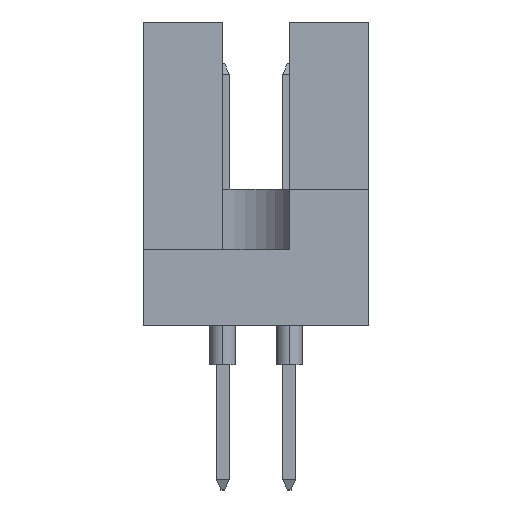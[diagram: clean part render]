
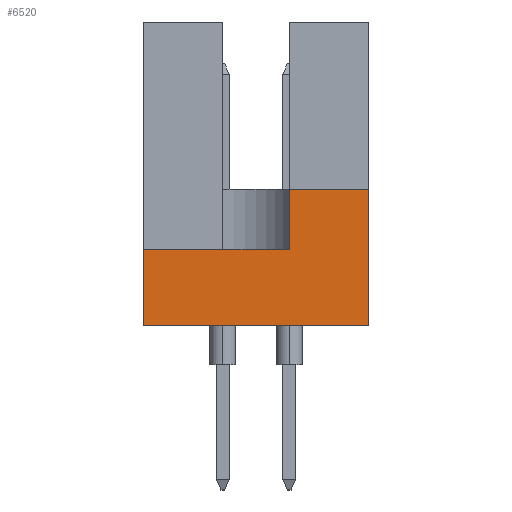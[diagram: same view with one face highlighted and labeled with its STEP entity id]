
A CAD part, left-side view. The second image highlights one B-rep face of the part: STEP entity #6520.
In plain terms, the highlighted planar face has unit normal (-1, 0, 0).
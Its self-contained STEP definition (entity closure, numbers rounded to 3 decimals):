
#75 = LINE ( 'NONE', #5244, #7016 ) ;
#217 = CARTESIAN_POINT ( 'NONE',  ( -47.5, -1.27, 2.9 ) ) ;
#599 = CARTESIAN_POINT ( 'NONE',  ( -47.5, -1.27, 19.02 ) ) ;
#619 = VECTOR ( 'NONE', #12354, 1000. ) ;
#737 = EDGE_LOOP ( 'NONE', ( #1978, #6213, #4580, #10751, #9131, #5655 ) ) ;
#951 = EDGE_CURVE ( 'NONE', #4590, #9276, #6410, .T. ) ;
#1071 = CARTESIAN_POINT ( 'NONE',  ( -47.5, 4.3, 0. ) ) ;
#1280 = DIRECTION ( 'NONE',  ( 1., 0., 0. ) ) ;
#1549 = LINE ( 'NONE', #3487, #9352 ) ;
#1978 = ORIENTED_EDGE ( 'NONE', *, *, #951, .F. ) ;
#2092 = PLANE ( 'NONE',  #5794 ) ;
#2777 = VECTOR ( 'NONE', #7641, 1000. ) ;
#3355 = DIRECTION ( 'NONE',  ( 0., 0., -1. ) ) ;
#3487 = CARTESIAN_POINT ( 'NONE',  ( -47.5, 4.3, 11.6 ) ) ;
#3809 = CARTESIAN_POINT ( 'NONE',  ( -47.5, -4.3, 5.2 ) ) ;
#4474 = DIRECTION ( 'NONE',  ( 0., 0., -1. ) ) ;
#4580 = ORIENTED_EDGE ( 'NONE', *, *, #7950, .T. ) ;
#4590 = VERTEX_POINT ( 'NONE', #7019 ) ;
#4821 = CARTESIAN_POINT ( 'NONE',  ( -47.5, -4.3, 0. ) ) ;
#5093 = EDGE_CURVE ( 'NONE', #9420, #11876, #5805, .T. ) ;
#5109 = VECTOR ( 'NONE', #11801, 1000. ) ;
#5244 = CARTESIAN_POINT ( 'NONE',  ( -47.5, 4.3, 2.9 ) ) ;
#5418 = EDGE_CURVE ( 'NONE', #10398, #9420, #1549, .T. ) ;
#5422 = DIRECTION ( 'NONE',  ( 0., -1., 0. ) ) ;
#5504 = LINE ( 'NONE', #9497, #619 ) ;
#5655 = ORIENTED_EDGE ( 'NONE', *, *, #10116, .F. ) ;
#5794 = AXIS2_PLACEMENT_3D ( 'NONE', #11386, #1280, #3355 ) ;
#5805 = LINE ( 'NONE', #6873, #5109 ) ;
#6213 = ORIENTED_EDGE ( 'NONE', *, *, #8331, .T. ) ;
#6410 = LINE ( 'NONE', #12676, #6683 ) ;
#6520 = ADVANCED_FACE ( 'NONE', ( #7198 ), #2092, .F. ) ;
#6683 = VECTOR ( 'NONE', #5422, 1000. ) ;
#6873 = CARTESIAN_POINT ( 'NONE',  ( -47.5, 4.3, 0. ) ) ;
#6984 = DIRECTION ( 'NONE',  ( 0., 1., 0. ) ) ;
#7016 = VECTOR ( 'NONE', #6984, 1000. ) ;
#7019 = CARTESIAN_POINT ( 'NONE',  ( -47.5, -1.27, 5.2 ) ) ;
#7198 = FACE_OUTER_BOUND ( 'NONE', #737, .T. ) ;
#7641 = DIRECTION ( 'NONE',  ( 0., 0., -1. ) ) ;
#7950 = EDGE_CURVE ( 'NONE', #9040, #10398, #75, .T. ) ;
#8151 = CARTESIAN_POINT ( 'NONE',  ( -47.5, 4.3, 2.9 ) ) ;
#8331 = EDGE_CURVE ( 'NONE', #4590, #9040, #9835, .T. ) ;
#9040 = VERTEX_POINT ( 'NONE', #217 ) ;
#9131 = ORIENTED_EDGE ( 'NONE', *, *, #5093, .T. ) ;
#9276 = VERTEX_POINT ( 'NONE', #3809 ) ;
#9352 = VECTOR ( 'NONE', #4474, 1000. ) ;
#9420 = VERTEX_POINT ( 'NONE', #1071 ) ;
#9497 = CARTESIAN_POINT ( 'NONE',  ( -47.5, -4.3, 11.6 ) ) ;
#9835 = LINE ( 'NONE', #599, #2777 ) ;
#10116 = EDGE_CURVE ( 'NONE', #9276, #11876, #5504, .T. ) ;
#10398 = VERTEX_POINT ( 'NONE', #8151 ) ;
#10751 = ORIENTED_EDGE ( 'NONE', *, *, #5418, .T. ) ;
#11386 = CARTESIAN_POINT ( 'NONE',  ( -47.5, 4.3, 11.6 ) ) ;
#11801 = DIRECTION ( 'NONE',  ( 0., -1., 0. ) ) ;
#11876 = VERTEX_POINT ( 'NONE', #4821 ) ;
#12354 = DIRECTION ( 'NONE',  ( 0., 0., -1. ) ) ;
#12676 = CARTESIAN_POINT ( 'NONE',  ( -47.5, 4.3, 5.2 ) ) ;
